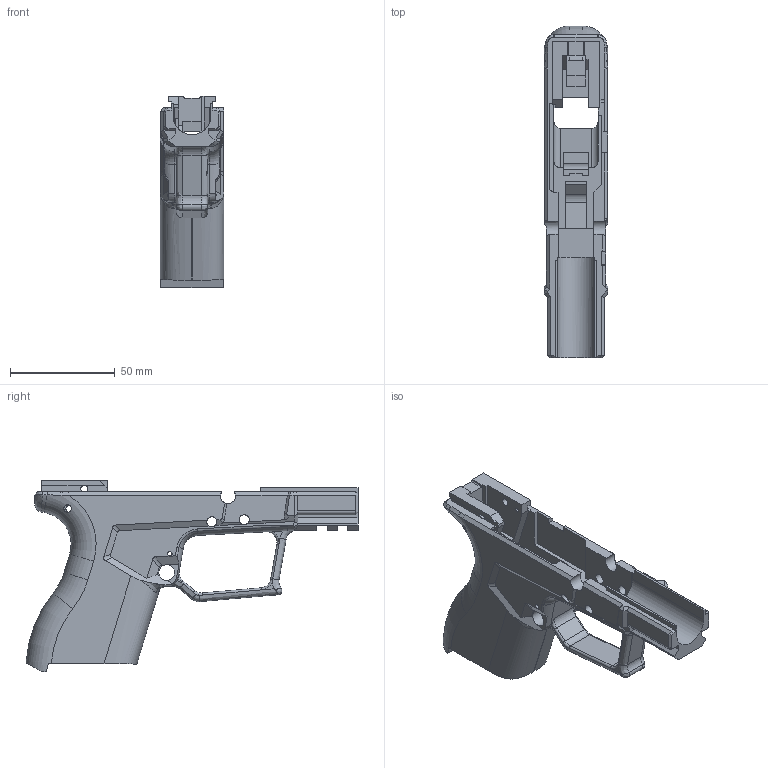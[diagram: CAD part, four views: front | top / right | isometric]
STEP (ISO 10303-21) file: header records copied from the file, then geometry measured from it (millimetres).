
FILE_DESCRIPTION(/* description */ (''),/* implementation_level */ '2;1');
FILE_NAME(/* name */ 'XD_subcompact v11 2_25_2022 v1.step',/* time_stamp */ '2022-03-30T22:27:37-04:00',/* author */ (''),/* organization */ (''),/* preprocessor_version */ 'ST-DEVELOPER v18.1',/* originating_system */ 'Autodesk Translation Framework v10.13.0.1454',/* authorisation */ '');
FILE_SCHEMA (('AUTOMOTIVE_DESIGN { 1 0 10303 214 3 1 1 }'));
Length unit declared in the file: millimetre
Products named in the file (1): XD_subcompact v11 2_25_2022
Bounding box: 30.25 x 158.31 x 91.2 mm (x, y, z)
Volume: 82739.9 mm3; surface area: 39806.3 mm2
Topology: 1 solids, 1 shells, 353 faces, 1013 edges, 642 vertices
Faces by surface type: plane 208, cylinder 73, bspline 50, torus 18, cone 4
Full cylindrical faces by diameter (mm): 1.9 x1, 2.15 x2, 3.4 x2, 3.54 x2, 4.76 x2, 4.8 x1, 4.9 x1, 7.5 x1
Entity records: 15361 total; most frequent: CARTESIAN_POINT 6196, ORIENTED_EDGE 2022, DIRECTION 1777, EDGE_CURVE 1011, LINE 655, VECTOR 655, VERTEX_POINT 642, AXIS2_PLACEMENT_3D 561
